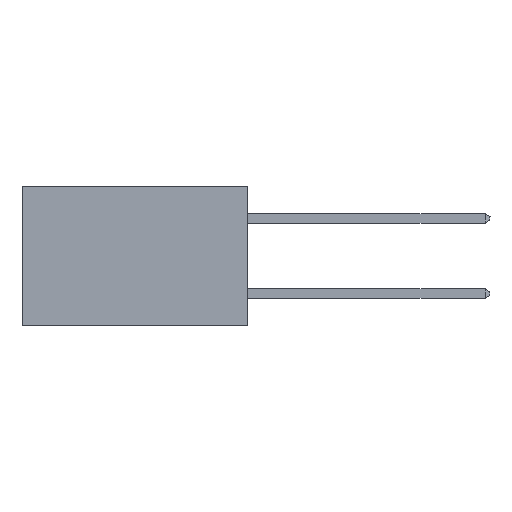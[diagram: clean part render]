
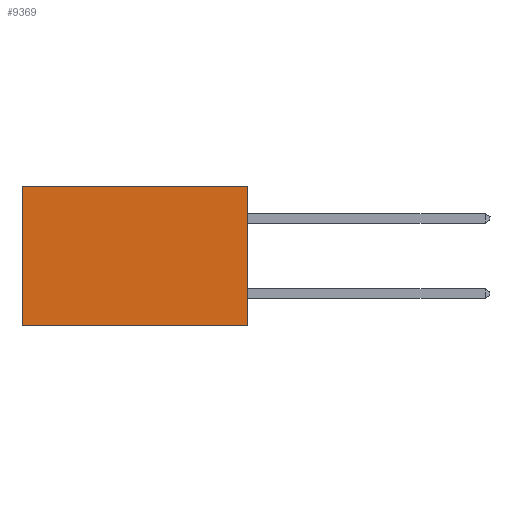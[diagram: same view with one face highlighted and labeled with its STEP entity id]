
A CAD part, left-side view. The second image highlights one B-rep face of the part: STEP entity #9369.
In plain terms, the highlighted planar face has unit normal (-1, 0, 0).
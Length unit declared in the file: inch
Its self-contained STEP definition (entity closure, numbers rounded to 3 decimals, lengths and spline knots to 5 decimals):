
#191 = CARTESIAN_POINT ( 'NONE',  ( 0.298, 0.6, 0. ) ) ;
#318 = ORIENTED_EDGE ( 'NONE', *, *, #5058, .F. ) ;
#1856 = ORIENTED_EDGE ( 'NONE', *, *, #19366, .T. ) ;
#3119 = LINE ( 'NONE', #191, #23683 ) ;
#3810 = CARTESIAN_POINT ( 'NONE',  ( 0.298, 0., 0. ) ) ;
#5058 = EDGE_CURVE ( 'NONE', #24786, #11019, #5570, .T. ) ;
#5570 = LINE ( 'NONE', #10638, #12252 ) ;
#5576 = CARTESIAN_POINT ( 'NONE',  ( 0.298, 0.6, -0.37 ) ) ;
#5844 = DIRECTION ( 'NONE',  ( 0., 1., 0. ) ) ;
#6452 = DIRECTION ( 'NONE',  ( 0., 0., -1. ) ) ;
#7267 = ORIENTED_EDGE ( 'NONE', *, *, #16552, .F. ) ;
#7956 = PLANE ( 'NONE',  #8056 ) ;
#8056 = AXIS2_PLACEMENT_3D ( 'NONE', #3810, #12018, #25664 ) ;
#9295 = CARTESIAN_POINT ( 'NONE',  ( 0.298, 0.6, 0. ) ) ;
#9369 = ADVANCED_FACE ( 'NONE', ( #18869 ), #7956, .F. ) ;
#9424 = LINE ( 'NONE', #19057, #13511 ) ;
#10610 = VERTEX_POINT ( 'NONE', #24198 ) ;
#10638 = CARTESIAN_POINT ( 'NONE',  ( 0.298, 0., -0.37 ) ) ;
#11019 = VERTEX_POINT ( 'NONE', #5576 ) ;
#12018 = DIRECTION ( 'NONE',  ( 1., 0., 0. ) ) ;
#12252 = VECTOR ( 'NONE', #19759, 39.37008 ) ;
#12589 = EDGE_LOOP ( 'NONE', ( #25428, #318, #7267, #1856 ) ) ;
#13238 = CARTESIAN_POINT ( 'NONE',  ( 0.298, 0., -0.37 ) ) ;
#13511 = VECTOR ( 'NONE', #24886, 39.37008 ) ;
#13671 = LINE ( 'NONE', #21741, #24968 ) ;
#16552 = EDGE_CURVE ( 'NONE', #10610, #24786, #9424, .T. ) ;
#18869 = FACE_OUTER_BOUND ( 'NONE', #12589, .T. ) ;
#19057 = CARTESIAN_POINT ( 'NONE',  ( 0.298, 0., 0. ) ) ;
#19366 = EDGE_CURVE ( 'NONE', #10610, #22336, #13671, .T. ) ;
#19759 = DIRECTION ( 'NONE',  ( 0., 1., 0. ) ) ;
#20806 = EDGE_CURVE ( 'NONE', #22336, #11019, #3119, .T. ) ;
#21741 = CARTESIAN_POINT ( 'NONE',  ( 0.298, 0., 0. ) ) ;
#22336 = VERTEX_POINT ( 'NONE', #9295 ) ;
#23683 = VECTOR ( 'NONE', #6452, 39.37008 ) ;
#24198 = CARTESIAN_POINT ( 'NONE',  ( 0.298, 0., 0. ) ) ;
#24786 = VERTEX_POINT ( 'NONE', #13238 ) ;
#24886 = DIRECTION ( 'NONE',  ( 0., 0., -1. ) ) ;
#24968 = VECTOR ( 'NONE', #5844, 39.37008 ) ;
#25428 = ORIENTED_EDGE ( 'NONE', *, *, #20806, .T. ) ;
#25664 = DIRECTION ( 'NONE',  ( 0., 0., -1. ) ) ;
